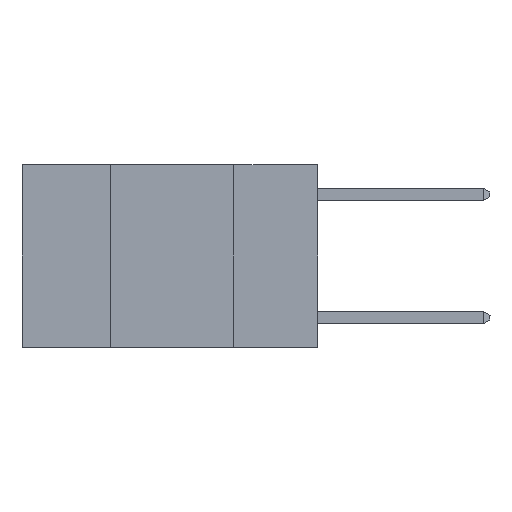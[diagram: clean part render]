
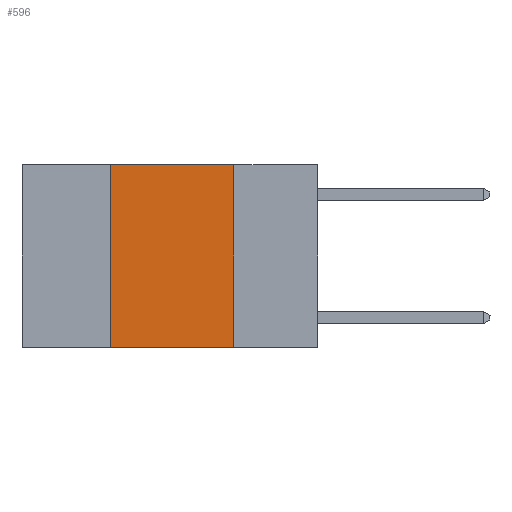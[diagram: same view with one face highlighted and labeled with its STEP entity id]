
A CAD part, left-side view. The second image highlights one B-rep face of the part: STEP entity #596.
In plain terms, the highlighted planar face has unit normal (-1, 0, 0).
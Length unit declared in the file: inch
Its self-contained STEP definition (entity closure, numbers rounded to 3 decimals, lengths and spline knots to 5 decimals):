
#53 = LINE ( 'NONE', #1200, #6975 ) ;
#128 = CARTESIAN_POINT ( 'NONE',  ( 0., 0.42, 0. ) ) ;
#595 = DIRECTION ( 'NONE',  ( 0., 0., 1. ) ) ;
#596 = ADVANCED_FACE ( 'NONE', ( #8096 ), #7438, .F. ) ;
#659 = VERTEX_POINT ( 'NONE', #6019 ) ;
#1200 = CARTESIAN_POINT ( 'NONE',  ( 0., 0.42, 0. ) ) ;
#1242 = VECTOR ( 'NONE', #6215, 39.37008 ) ;
#1478 = VERTEX_POINT ( 'NONE', #4107 ) ;
#1565 = ORIENTED_EDGE ( 'NONE', *, *, #4622, .F. ) ;
#1653 = DIRECTION ( 'NONE',  ( 1., 0., 0. ) ) ;
#1790 = CARTESIAN_POINT ( 'NONE',  ( 0., 0.6, -0.37 ) ) ;
#1810 = DIRECTION ( 'NONE',  ( 0., -1., 0. ) ) ;
#2260 = EDGE_CURVE ( 'NONE', #1478, #4248, #53, .T. ) ;
#2556 = EDGE_CURVE ( 'NONE', #1478, #659, #3475, .T. ) ;
#2966 = DIRECTION ( 'NONE',  ( 0., 0., -1. ) ) ;
#3227 = VERTEX_POINT ( 'NONE', #4895 ) ;
#3268 = VECTOR ( 'NONE', #1810, 39.37008 ) ;
#3475 = LINE ( 'NONE', #1790, #3268 ) ;
#3520 = VECTOR ( 'NONE', #7604, 39.37008 ) ;
#3811 = ORIENTED_EDGE ( 'NONE', *, *, #2556, .T. ) ;
#3951 = CARTESIAN_POINT ( 'NONE',  ( 0., 0.6, 0. ) ) ;
#4107 = CARTESIAN_POINT ( 'NONE',  ( 0., 0.42, -0.37 ) ) ;
#4248 = VERTEX_POINT ( 'NONE', #128 ) ;
#4276 = AXIS2_PLACEMENT_3D ( 'NONE', #3951, #1653, #2966 ) ;
#4349 = ORIENTED_EDGE ( 'NONE', *, *, #2260, .F. ) ;
#4622 = EDGE_CURVE ( 'NONE', #3227, #659, #7307, .T. ) ;
#4895 = CARTESIAN_POINT ( 'NONE',  ( 0., 0.17, 0. ) ) ;
#5069 = CARTESIAN_POINT ( 'NONE',  ( 0., 0.17, 0. ) ) ;
#6019 = CARTESIAN_POINT ( 'NONE',  ( 0., 0.17, -0.37 ) ) ;
#6215 = DIRECTION ( 'NONE',  ( 0., -1., 0. ) ) ;
#6345 = ORIENTED_EDGE ( 'NONE', *, *, #8226, .F. ) ;
#6427 = LINE ( 'NONE', #6815, #1242 ) ;
#6815 = CARTESIAN_POINT ( 'NONE',  ( 0., 0.6, 0. ) ) ;
#6975 = VECTOR ( 'NONE', #595, 39.37008 ) ;
#7307 = LINE ( 'NONE', #5069, #3520 ) ;
#7438 = PLANE ( 'NONE',  #4276 ) ;
#7604 = DIRECTION ( 'NONE',  ( 0., 0., -1. ) ) ;
#7690 = EDGE_LOOP ( 'NONE', ( #1565, #6345, #4349, #3811 ) ) ;
#8096 = FACE_OUTER_BOUND ( 'NONE', #7690, .T. ) ;
#8226 = EDGE_CURVE ( 'NONE', #4248, #3227, #6427, .T. ) ;
